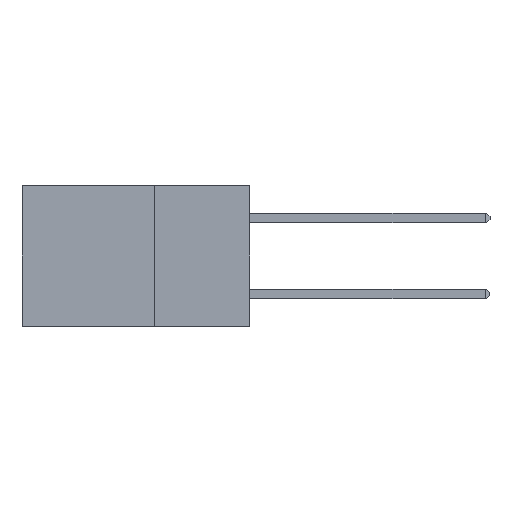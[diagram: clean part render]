
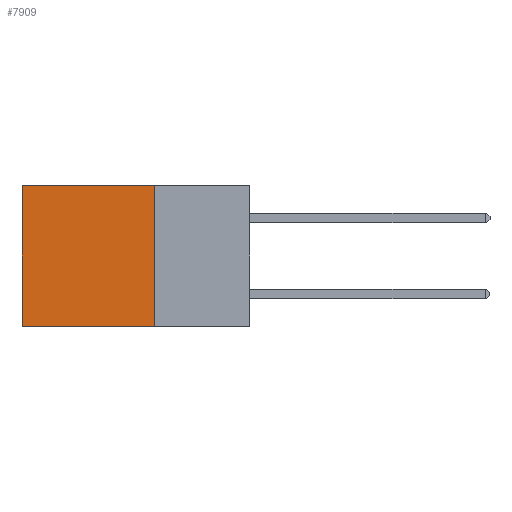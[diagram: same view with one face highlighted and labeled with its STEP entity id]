
A CAD part, left-side view. The second image highlights one B-rep face of the part: STEP entity #7909.
In plain terms, the highlighted planar face has unit normal (-1, 0, 0).
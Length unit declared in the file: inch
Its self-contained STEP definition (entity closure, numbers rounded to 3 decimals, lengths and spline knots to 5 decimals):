
#52 = CARTESIAN_POINT ( 'NONE',  ( 0.2875, 0.25, 0. ) ) ;
#404 = ORIENTED_EDGE ( 'NONE', *, *, #11754, .F. ) ;
#827 = ORIENTED_EDGE ( 'NONE', *, *, #4558, .F. ) ;
#1340 = DIRECTION ( 'NONE',  ( 0., 0., -1. ) ) ;
#2051 = CARTESIAN_POINT ( 'NONE',  ( 0.2875, 0.6, -0.37 ) ) ;
#2176 = LINE ( 'NONE', #12230, #8452 ) ;
#2257 = EDGE_LOOP ( 'NONE', ( #13224, #827, #404, #2878 ) ) ;
#2336 = LINE ( 'NONE', #4808, #8234 ) ;
#2463 = CARTESIAN_POINT ( 'NONE',  ( 0.2875, 0.25, 0. ) ) ;
#2878 = ORIENTED_EDGE ( 'NONE', *, *, #13309, .T. ) ;
#3950 = VERTEX_POINT ( 'NONE', #7124 ) ;
#4470 = DIRECTION ( 'NONE',  ( 0., 1., 0. ) ) ;
#4553 = DIRECTION ( 'NONE',  ( 0., 1., 0. ) ) ;
#4558 = EDGE_CURVE ( 'NONE', #10319, #12844, #13145, .T. ) ;
#4575 = LINE ( 'NONE', #10597, #7852 ) ;
#4808 = CARTESIAN_POINT ( 'NONE',  ( 0.2875, 0.6, 0. ) ) ;
#5706 = CARTESIAN_POINT ( 'NONE',  ( 0.2875, 0.25, -0.37 ) ) ;
#6446 = PLANE ( 'NONE',  #6892 ) ;
#6892 = AXIS2_PLACEMENT_3D ( 'NONE', #52, #8884, #1340 ) ;
#7124 = CARTESIAN_POINT ( 'NONE',  ( 0.2875, 0.6, 0. ) ) ;
#7735 = EDGE_CURVE ( 'NONE', #3950, #12844, #2336, .T. ) ;
#7852 = VECTOR ( 'NONE', #4553, 39.37008 ) ;
#7909 = ADVANCED_FACE ( 'NONE', ( #11944 ), #6446, .F. ) ;
#8234 = VECTOR ( 'NONE', #10907, 39.37008 ) ;
#8452 = VECTOR ( 'NONE', #13429, 39.37008 ) ;
#8884 = DIRECTION ( 'NONE',  ( 1., 0., 0. ) ) ;
#10319 = VERTEX_POINT ( 'NONE', #5706 ) ;
#10597 = CARTESIAN_POINT ( 'NONE',  ( 0.2875, 0.25, 0. ) ) ;
#10907 = DIRECTION ( 'NONE',  ( 0., 0., -1. ) ) ;
#11754 = EDGE_CURVE ( 'NONE', #14196, #10319, #2176, .T. ) ;
#11944 = FACE_OUTER_BOUND ( 'NONE', #2257, .T. ) ;
#12230 = CARTESIAN_POINT ( 'NONE',  ( 0.2875, 0.25, 0. ) ) ;
#12777 = VECTOR ( 'NONE', #4470, 39.37008 ) ;
#12844 = VERTEX_POINT ( 'NONE', #2051 ) ;
#12903 = CARTESIAN_POINT ( 'NONE',  ( 0.2875, 0.25, -0.37 ) ) ;
#13145 = LINE ( 'NONE', #12903, #12777 ) ;
#13224 = ORIENTED_EDGE ( 'NONE', *, *, #7735, .T. ) ;
#13309 = EDGE_CURVE ( 'NONE', #14196, #3950, #4575, .T. ) ;
#13429 = DIRECTION ( 'NONE',  ( 0., 0., -1. ) ) ;
#14196 = VERTEX_POINT ( 'NONE', #2463 ) ;
